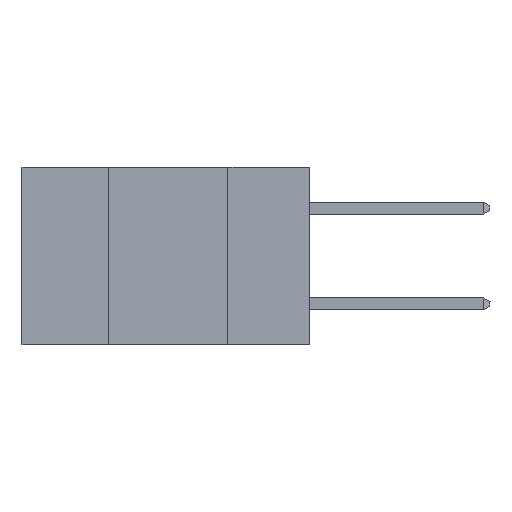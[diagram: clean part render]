
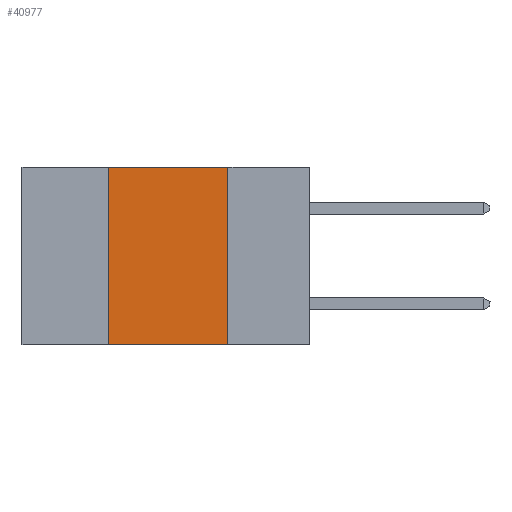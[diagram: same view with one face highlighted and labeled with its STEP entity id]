
A CAD part, left-side view. The second image highlights one B-rep face of the part: STEP entity #40977.
In plain terms, the highlighted planar face has unit normal (-1, 0, 0).
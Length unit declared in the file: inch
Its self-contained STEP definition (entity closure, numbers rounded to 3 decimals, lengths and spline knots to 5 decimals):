
#2498 = AXIS2_PLACEMENT_3D ( 'NONE', #16943, #37014, #7433 ) ;
#3571 = CARTESIAN_POINT ( 'NONE',  ( 0., 0.17, -0.37 ) ) ;
#5656 = EDGE_CURVE ( 'NONE', #25565, #22307, #28229, .T. ) ;
#7433 = DIRECTION ( 'NONE',  ( 0., 0., -1. ) ) ;
#7483 = VECTOR ( 'NONE', #8727, 39.37008 ) ;
#7693 = CARTESIAN_POINT ( 'NONE',  ( 0., 0.42, 0. ) ) ;
#8727 = DIRECTION ( 'NONE',  ( 0., -1., 0. ) ) ;
#9614 = ORIENTED_EDGE ( 'NONE', *, *, #21342, .F. ) ;
#11863 = DIRECTION ( 'NONE',  ( 0., 0., 1. ) ) ;
#14082 = EDGE_CURVE ( 'NONE', #22307, #36821, #18625, .T. ) ;
#14586 = CARTESIAN_POINT ( 'NONE',  ( 0., 0.17, 0. ) ) ;
#16798 = VECTOR ( 'NONE', #33914, 39.37008 ) ;
#16943 = CARTESIAN_POINT ( 'NONE',  ( 0., 0.6, 0. ) ) ;
#18625 = LINE ( 'NONE', #28541, #36423 ) ;
#20184 = PLANE ( 'NONE',  #2498 ) ;
#21342 = EDGE_CURVE ( 'NONE', #36821, #22762, #24608, .T. ) ;
#22307 = VERTEX_POINT ( 'NONE', #7693 ) ;
#22762 = VERTEX_POINT ( 'NONE', #3571 ) ;
#24608 = LINE ( 'NONE', #34331, #16798 ) ;
#24804 = VECTOR ( 'NONE', #11863, 39.37008 ) ;
#25199 = ORIENTED_EDGE ( 'NONE', *, *, #33510, .T. ) ;
#25565 = VERTEX_POINT ( 'NONE', #37137 ) ;
#28229 = LINE ( 'NONE', #41430, #24804 ) ;
#28541 = CARTESIAN_POINT ( 'NONE',  ( 0., 0.6, 0. ) ) ;
#33510 = EDGE_CURVE ( 'NONE', #25565, #22762, #39140, .T. ) ;
#33914 = DIRECTION ( 'NONE',  ( 0., 0., -1. ) ) ;
#34331 = CARTESIAN_POINT ( 'NONE',  ( 0., 0.17, 0. ) ) ;
#36423 = VECTOR ( 'NONE', #38926, 39.37008 ) ;
#36821 = VERTEX_POINT ( 'NONE', #14586 ) ;
#37014 = DIRECTION ( 'NONE',  ( 1., 0., 0. ) ) ;
#37137 = CARTESIAN_POINT ( 'NONE',  ( 0., 0.42, -0.37 ) ) ;
#37227 = FACE_OUTER_BOUND ( 'NONE', #41790, .T. ) ;
#38926 = DIRECTION ( 'NONE',  ( 0., -1., 0. ) ) ;
#39140 = LINE ( 'NONE', #42403, #7483 ) ;
#40405 = ORIENTED_EDGE ( 'NONE', *, *, #5656, .F. ) ;
#40977 = ADVANCED_FACE ( 'NONE', ( #37227 ), #20184, .F. ) ;
#41430 = CARTESIAN_POINT ( 'NONE',  ( 0., 0.42, 0. ) ) ;
#41790 = EDGE_LOOP ( 'NONE', ( #9614, #42629, #40405, #25199 ) ) ;
#42403 = CARTESIAN_POINT ( 'NONE',  ( 0., 0.6, -0.37 ) ) ;
#42629 = ORIENTED_EDGE ( 'NONE', *, *, #14082, .F. ) ;
